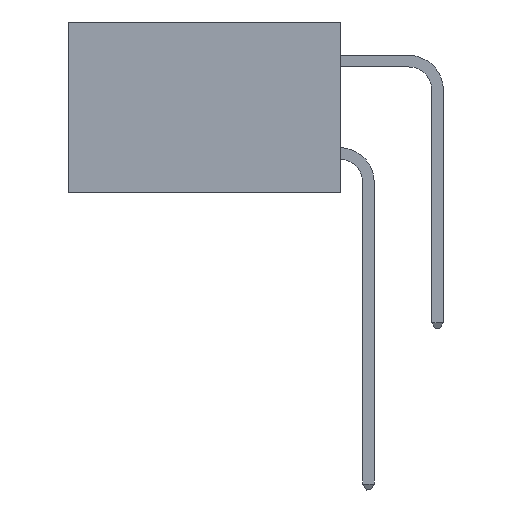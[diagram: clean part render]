
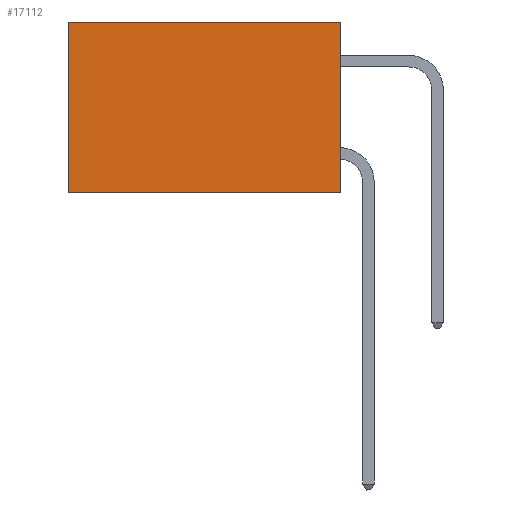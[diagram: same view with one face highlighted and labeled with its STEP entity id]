
A CAD part, left-side view. The second image highlights one B-rep face of the part: STEP entity #17112.
In plain terms, the highlighted planar face has unit normal (-1, 0, 0).
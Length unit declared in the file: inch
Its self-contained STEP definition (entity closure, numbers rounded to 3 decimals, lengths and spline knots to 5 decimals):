
#752 = CARTESIAN_POINT ( 'NONE',  ( 0.277, 0., -0.37 ) ) ;
#1288 = EDGE_LOOP ( 'NONE', ( #1746, #17843, #22078, #22822 ) ) ;
#1746 = ORIENTED_EDGE ( 'NONE', *, *, #27413, .T. ) ;
#3016 = EDGE_CURVE ( 'NONE', #28122, #15348, #8326, .T. ) ;
#3564 = PLANE ( 'NONE',  #29053 ) ;
#4726 = VECTOR ( 'NONE', #20290, 39.37008 ) ;
#5008 = EDGE_CURVE ( 'NONE', #19022, #28122, #19283, .T. ) ;
#5584 = LINE ( 'NONE', #9425, #4726 ) ;
#6100 = CARTESIAN_POINT ( 'NONE',  ( 0.277, 0.59, -0.37 ) ) ;
#6324 = DIRECTION ( 'NONE',  ( 1., 0., 0. ) ) ;
#7005 = VERTEX_POINT ( 'NONE', #29230 ) ;
#8326 = LINE ( 'NONE', #27348, #29162 ) ;
#8541 = FACE_OUTER_BOUND ( 'NONE', #1288, .T. ) ;
#9425 = CARTESIAN_POINT ( 'NONE',  ( 0.277, 0., 0. ) ) ;
#13950 = CARTESIAN_POINT ( 'NONE',  ( 0.277, 0., 0. ) ) ;
#15348 = VERTEX_POINT ( 'NONE', #16210 ) ;
#16210 = CARTESIAN_POINT ( 'NONE',  ( 0.277, 0.59, -0.37 ) ) ;
#17112 = ADVANCED_FACE ( 'NONE', ( #8541 ), #3564, .F. ) ;
#17843 = ORIENTED_EDGE ( 'NONE', *, *, #3016, .F. ) ;
#19022 = VERTEX_POINT ( 'NONE', #13950 ) ;
#19283 = LINE ( 'NONE', #26057, #32787 ) ;
#19908 = CARTESIAN_POINT ( 'NONE',  ( 0.277, 0., -0.37 ) ) ;
#20290 = DIRECTION ( 'NONE',  ( 0., 1., 0. ) ) ;
#22078 = ORIENTED_EDGE ( 'NONE', *, *, #5008, .F. ) ;
#22439 = DIRECTION ( 'NONE',  ( 0., 0., -1. ) ) ;
#22822 = ORIENTED_EDGE ( 'NONE', *, *, #27004, .T. ) ;
#25385 = DIRECTION ( 'NONE',  ( 0., 0., -1. ) ) ;
#25557 = DIRECTION ( 'NONE',  ( 0., 0., -1. ) ) ;
#26057 = CARTESIAN_POINT ( 'NONE',  ( 0.277, 0., -0.37 ) ) ;
#26465 = VECTOR ( 'NONE', #22439, 39.37008 ) ;
#27004 = EDGE_CURVE ( 'NONE', #19022, #7005, #5584, .T. ) ;
#27348 = CARTESIAN_POINT ( 'NONE',  ( 0.277, 0., -0.37 ) ) ;
#27413 = EDGE_CURVE ( 'NONE', #7005, #15348, #33541, .T. ) ;
#28122 = VERTEX_POINT ( 'NONE', #752 ) ;
#29053 = AXIS2_PLACEMENT_3D ( 'NONE', #19908, #6324, #25385 ) ;
#29162 = VECTOR ( 'NONE', #34440, 39.37008 ) ;
#29230 = CARTESIAN_POINT ( 'NONE',  ( 0.277, 0.59, 0. ) ) ;
#32787 = VECTOR ( 'NONE', #25557, 39.37008 ) ;
#33541 = LINE ( 'NONE', #6100, #26465 ) ;
#34440 = DIRECTION ( 'NONE',  ( 0., 1., 0. ) ) ;
